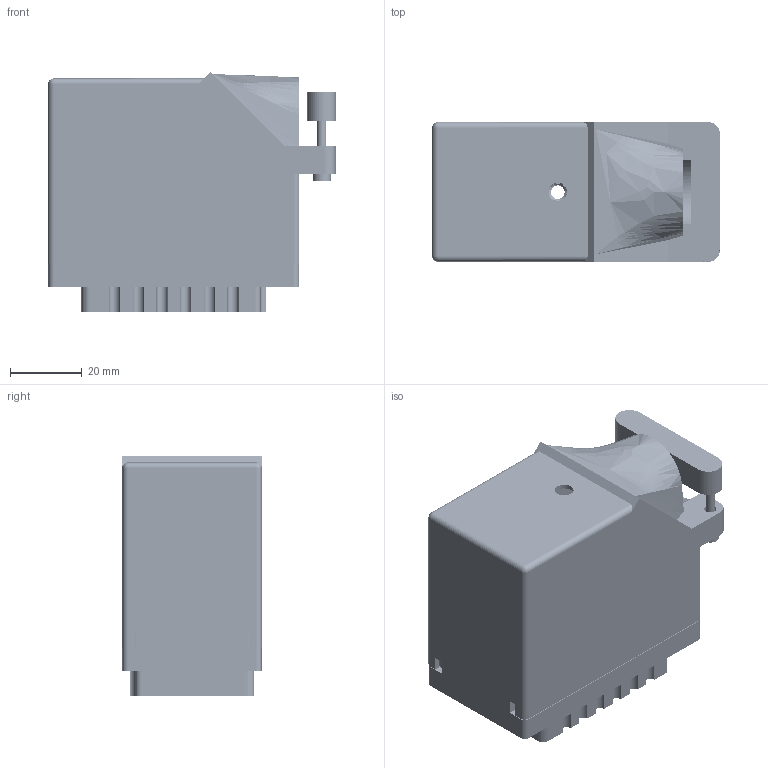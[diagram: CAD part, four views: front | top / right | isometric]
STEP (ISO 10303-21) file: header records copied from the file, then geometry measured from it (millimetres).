
FILE_DESCRIPTION (( 'STEP AP203' ), '1' );
FILE_NAME ('516-120-500-426.STEP', '2020-03-07T00:54:17', ( '' ), ( '' ), 'SwSTEP 2.0', 'SolidWorks 2016', '' );
FILE_SCHEMA (( 'CONFIG_CONTROL_DESIGN' ));
Length unit declared in the file: inch
Products named in the file (5): 516-292-001_500 Contact; 516-120-500-426; 516 Part Receptacle_120; 516-230-001_Plastic - 120 Side Entry; 516-252-095-100
Assembly tree (123 placements, depth 2):
  516-120-500-426
    516 Part Receptacle_120
    516-292-001_500 Contact  x120
    516-230-001_Plastic - 120 Side Entry
    516-252-095-100
Bounding box: 80.14 x 38.86 x 66.85 mm (x, y, z)
Volume: 52047 mm3; surface area: 87446.8 mm2
Topology: 123 solids, 123 shells, 11728 faces, 34121 edges, 22661 vertices
Faces by surface type: plane 6999, cylinder 3986, bspline 729, cone 12, sphere 2
Entity records: 96697 total; most frequent: CARTESIAN_POINT 18426, ORIENTED_EDGE 15878, DIRECTION 15451, EDGE_CURVE 7939, VECTOR 5845, LINE 5845, VERTEX_POINT 5287, AXIS2_PLACEMENT_3D 4803
